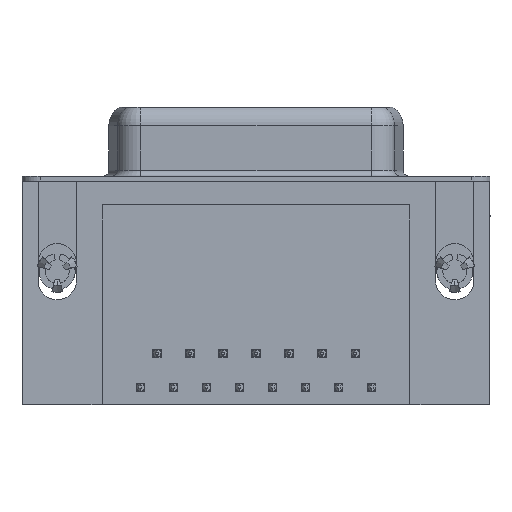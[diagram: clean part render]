
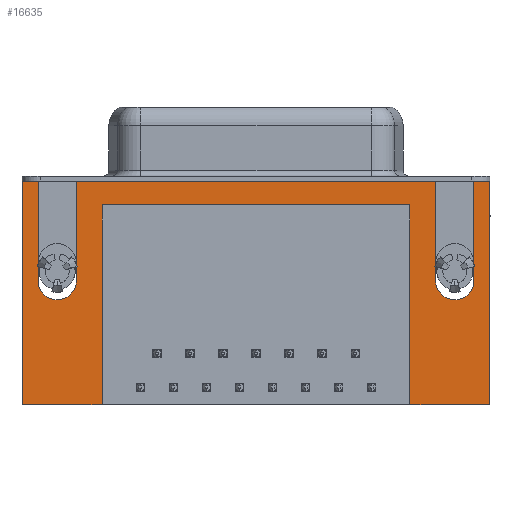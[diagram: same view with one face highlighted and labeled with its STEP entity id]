
A CAD part, front view. The second image highlights one B-rep face of the part: STEP entity #16635.
In plain terms, the highlighted planar face has unit normal (0, -1, 0).
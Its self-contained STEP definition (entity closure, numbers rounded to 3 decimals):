
#9 = ORIENTED_EDGE ( 'NONE', *, *, #11276, .F. ) ;
#13 = ORIENTED_EDGE ( 'NONE', *, *, #11727, .F. ) ;
#138 = EDGE_CURVE ( 'NONE', #19946, #1787, #15826, .T. ) ;
#284 = AXIS2_PLACEMENT_3D ( 'NONE', #16325, #4388, #18407 ) ;
#1061 = EDGE_CURVE ( 'NONE', #15841, #18148, #12782, .T. ) ;
#1199 = VERTEX_POINT ( 'NONE', #4365 ) ;
#1600 = VERTEX_POINT ( 'NONE', #13867 ) ;
#1777 = EDGE_CURVE ( 'NONE', #19913, #17454, #9940, .T. ) ;
#1787 = VERTEX_POINT ( 'NONE', #24014 ) ;
#1871 = DIRECTION ( 'NONE',  ( 0., 0., 1. ) ) ;
#1970 = DIRECTION ( 'NONE',  ( -1., 0., 0. ) ) ;
#2057 = CARTESIAN_POINT ( 'NONE',  ( 1.6, -6.275, -8.35 ) ) ;
#2723 = VERTEX_POINT ( 'NONE', #14955 ) ;
#2926 = DIRECTION ( 'NONE',  ( 0., 0., -1. ) ) ;
#3282 = CARTESIAN_POINT ( 'NONE',  ( -2.935, -6.275, -2.5 ) ) ;
#3565 = DIRECTION ( 'NONE',  ( 0., 0., 1. ) ) ;
#3610 = PLANE ( 'NONE',  #19055 ) ;
#3682 = LINE ( 'NONE', #25993, #3729 ) ;
#3729 = VECTOR ( 'NONE', #1970, 1000. ) ;
#3879 = VECTOR ( 'NONE', #3565, 1000. ) ;
#3900 = LINE ( 'NONE', #19445, #3879 ) ;
#4109 = CARTESIAN_POINT ( 'NONE',  ( 36.255, -6.275, -2.5 ) ) ;
#4287 = VECTOR ( 'NONE', #22861, 1000. ) ;
#4332 = LINE ( 'NONE', #4959, #4287 ) ;
#4365 = CARTESIAN_POINT ( 'NONE',  ( 3.765, -6.275, -18.76 ) ) ;
#4388 = DIRECTION ( 'NONE',  ( 0., -1., 0. ) ) ;
#4413 = DIRECTION ( 'NONE',  ( 0., -1., 0. ) ) ;
#4959 = CARTESIAN_POINT ( 'NONE',  ( 3.765, -6.275, -2. ) ) ;
#5014 = VECTOR ( 'NONE', #18012, 1000. ) ;
#5252 = LINE ( 'NONE', #23965, #5014 ) ;
#5380 = ORIENTED_EDGE ( 'NONE', *, *, #24785, .F. ) ;
#5638 = CARTESIAN_POINT ( 'NONE',  ( 3.765, -6.275, -2. ) ) ;
#5723 = LINE ( 'NONE', #21629, #6000 ) ;
#5856 = ORIENTED_EDGE ( 'NONE', *, *, #12225, .F. ) ;
#6000 = VECTOR ( 'NONE', #9597, 1000. ) ;
#6244 = LINE ( 'NONE', #24634, #6322 ) ;
#6322 = VECTOR ( 'NONE', #22693, 1000. ) ;
#6564 = CIRCLE ( 'NONE', #20812, 1.6 ) ;
#6579 = VECTOR ( 'NONE', #7808, 1000. ) ;
#6612 = ORIENTED_EDGE ( 'NONE', *, *, #10503, .F. ) ;
#6636 = LINE ( 'NONE', #25855, #6579 ) ;
#6927 = CARTESIAN_POINT ( 'NONE',  ( 31.72, -6.275, 0. ) ) ;
#7110 = LINE ( 'NONE', #6927, #7138 ) ;
#7138 = VECTOR ( 'NONE', #2926, 1000. ) ;
#7291 = DIRECTION ( 'NONE',  ( 0., 0., 1. ) ) ;
#7591 = CIRCLE ( 'NONE', #284, 1.6 ) ;
#7642 = CARTESIAN_POINT ( 'NONE',  ( -2.935, -6.275, -2.5 ) ) ;
#7808 = DIRECTION ( 'NONE',  ( 0., 0., 1. ) ) ;
#7851 = VERTEX_POINT ( 'NONE', #11373 ) ;
#8012 = VERTEX_POINT ( 'NONE', #2057 ) ;
#8105 = LINE ( 'NONE', #9827, #8156 ) ;
#8156 = VECTOR ( 'NONE', #1871, 1000. ) ;
#8493 = EDGE_CURVE ( 'NONE', #2723, #15841, #13875, .T. ) ;
#8685 = CARTESIAN_POINT ( 'NONE',  ( 31.72, -6.275, 0. ) ) ;
#8746 = CARTESIAN_POINT ( 'NONE',  ( 1.6, -6.275, 0. ) ) ;
#8886 = ORIENTED_EDGE ( 'NONE', *, *, #11459, .F. ) ;
#9414 = EDGE_CURVE ( 'NONE', #19443, #1787, #11046, .T. ) ;
#9597 = DIRECTION ( 'NONE',  ( -1., 0., 0. ) ) ;
#9819 = VECTOR ( 'NONE', #13187, 1000. ) ;
#9827 = CARTESIAN_POINT ( 'NONE',  ( 34.92, -6.275, 0. ) ) ;
#9940 = LINE ( 'NONE', #15405, #9819 ) ;
#10503 = EDGE_CURVE ( 'NONE', #14047, #19946, #8105, .T. ) ;
#10647 = ORIENTED_EDGE ( 'NONE', *, *, #9414, .T. ) ;
#10713 = EDGE_CURVE ( 'NONE', #19555, #14047, #7591, .T. ) ;
#10881 = EDGE_CURVE ( 'NONE', #17454, #19555, #7110, .T. ) ;
#11046 = LINE ( 'NONE', #4109, #11292 ) ;
#11113 = EDGE_CURVE ( 'NONE', #8012, #19913, #6636, .T. ) ;
#11276 = EDGE_CURVE ( 'NONE', #18148, #7851, #6244, .T. ) ;
#11292 = VECTOR ( 'NONE', #16024, 1000. ) ;
#11373 = CARTESIAN_POINT ( 'NONE',  ( -1.6, -6.275, -8.35 ) ) ;
#11459 = EDGE_CURVE ( 'NONE', #1199, #2723, #5723, .T. ) ;
#11585 = DIRECTION ( 'NONE',  ( 0., -1., 0. ) ) ;
#11727 = EDGE_CURVE ( 'NONE', #19646, #1199, #5252, .T. ) ;
#11913 = ORIENTED_EDGE ( 'NONE', *, *, #138, .F. ) ;
#11945 = EDGE_CURVE ( 'NONE', #1600, #19646, #4332, .T. ) ;
#12139 = EDGE_CURVE ( 'NONE', #23390, #1600, #3900, .T. ) ;
#12225 = EDGE_CURVE ( 'NONE', #19443, #23390, #3682, .T. ) ;
#12553 = VECTOR ( 'NONE', #19831, 1000. ) ;
#12782 = LINE ( 'NONE', #19663, #12553 ) ;
#13172 = CARTESIAN_POINT ( 'NONE',  ( 31.72, -6.275, -8.35 ) ) ;
#13187 = DIRECTION ( 'NONE',  ( 1., 0., 0. ) ) ;
#13630 = ORIENTED_EDGE ( 'NONE', *, *, #11113, .F. ) ;
#13726 = VECTOR ( 'NONE', #7291, 1000. ) ;
#13867 = CARTESIAN_POINT ( 'NONE',  ( 29.555, -6.275, -2. ) ) ;
#13875 = LINE ( 'NONE', #3282, #13726 ) ;
#13926 = CARTESIAN_POINT ( 'NONE',  ( -2.935, -6.275, 0. ) ) ;
#14047 = VERTEX_POINT ( 'NONE', #22217 ) ;
#14647 = FACE_OUTER_BOUND ( 'NONE', #18904, .T. ) ;
#14955 = CARTESIAN_POINT ( 'NONE',  ( -2.935, -6.275, -18.76 ) ) ;
#15326 = CARTESIAN_POINT ( 'NONE',  ( -1.6, -6.275, 0. ) ) ;
#15405 = CARTESIAN_POINT ( 'NONE',  ( -2.935, -6.275, 0. ) ) ;
#15749 = VECTOR ( 'NONE', #20457, 1000. ) ;
#15826 = LINE ( 'NONE', #13926, #15749 ) ;
#15841 = VERTEX_POINT ( 'NONE', #19640 ) ;
#16024 = DIRECTION ( 'NONE',  ( 0., 0., 1. ) ) ;
#16191 = ORIENTED_EDGE ( 'NONE', *, *, #1777, .F. ) ;
#16325 = CARTESIAN_POINT ( 'NONE',  ( 33.32, -6.275, -8.35 ) ) ;
#16347 = CARTESIAN_POINT ( 'NONE',  ( 0., -6.275, -8.35 ) ) ;
#16635 = ADVANCED_FACE ( 'NONE', ( #14647 ), #3610, .T. ) ;
#16780 = CARTESIAN_POINT ( 'NONE',  ( 34.92, -6.275, 0. ) ) ;
#17454 = VERTEX_POINT ( 'NONE', #8685 ) ;
#18012 = DIRECTION ( 'NONE',  ( 0., 0., -1. ) ) ;
#18148 = VERTEX_POINT ( 'NONE', #15326 ) ;
#18407 = DIRECTION ( 'NONE',  ( -1., 0., 0. ) ) ;
#18430 = DIRECTION ( 'NONE',  ( 1., 0., 0. ) ) ;
#18904 = EDGE_LOOP ( 'NONE', ( #6612, #19188, #22942, #16191, #13630, #5380, #9, #22566, #21232, #8886, #13, #21005, #20218, #5856, #10647, #11913 ) ) ;
#19055 = AXIS2_PLACEMENT_3D ( 'NONE', #7642, #11585, #25691 ) ;
#19188 = ORIENTED_EDGE ( 'NONE', *, *, #10713, .F. ) ;
#19443 = VERTEX_POINT ( 'NONE', #24926 ) ;
#19445 = CARTESIAN_POINT ( 'NONE',  ( 29.555, -6.275, -2. ) ) ;
#19555 = VERTEX_POINT ( 'NONE', #13172 ) ;
#19640 = CARTESIAN_POINT ( 'NONE',  ( -2.935, -6.275, 0. ) ) ;
#19646 = VERTEX_POINT ( 'NONE', #5638 ) ;
#19663 = CARTESIAN_POINT ( 'NONE',  ( -2.935, -6.275, 0. ) ) ;
#19831 = DIRECTION ( 'NONE',  ( 1., 0., 0. ) ) ;
#19913 = VERTEX_POINT ( 'NONE', #8746 ) ;
#19946 = VERTEX_POINT ( 'NONE', #16780 ) ;
#20218 = ORIENTED_EDGE ( 'NONE', *, *, #12139, .F. ) ;
#20457 = DIRECTION ( 'NONE',  ( 1., 0., 0. ) ) ;
#20812 = AXIS2_PLACEMENT_3D ( 'NONE', #16347, #4413, #18430 ) ;
#21005 = ORIENTED_EDGE ( 'NONE', *, *, #11945, .F. ) ;
#21232 = ORIENTED_EDGE ( 'NONE', *, *, #8493, .F. ) ;
#21629 = CARTESIAN_POINT ( 'NONE',  ( 36.255, -6.275, -18.76 ) ) ;
#22217 = CARTESIAN_POINT ( 'NONE',  ( 34.92, -6.275, -8.35 ) ) ;
#22566 = ORIENTED_EDGE ( 'NONE', *, *, #1061, .F. ) ;
#22693 = DIRECTION ( 'NONE',  ( 0., 0., -1. ) ) ;
#22861 = DIRECTION ( 'NONE',  ( -1., 0., 0. ) ) ;
#22942 = ORIENTED_EDGE ( 'NONE', *, *, #10881, .F. ) ;
#23240 = CARTESIAN_POINT ( 'NONE',  ( 29.555, -6.275, -18.76 ) ) ;
#23390 = VERTEX_POINT ( 'NONE', #23240 ) ;
#23965 = CARTESIAN_POINT ( 'NONE',  ( 3.765, -6.275, -2. ) ) ;
#24014 = CARTESIAN_POINT ( 'NONE',  ( 36.255, -6.275, 0. ) ) ;
#24634 = CARTESIAN_POINT ( 'NONE',  ( -1.6, -6.275, 0. ) ) ;
#24785 = EDGE_CURVE ( 'NONE', #7851, #8012, #6564, .T. ) ;
#24926 = CARTESIAN_POINT ( 'NONE',  ( 36.255, -6.275, -18.76 ) ) ;
#25691 = DIRECTION ( 'NONE',  ( 0., 0., -1. ) ) ;
#25855 = CARTESIAN_POINT ( 'NONE',  ( 1.6, -6.275, 0. ) ) ;
#25993 = CARTESIAN_POINT ( 'NONE',  ( 36.255, -6.275, -18.76 ) ) ;
